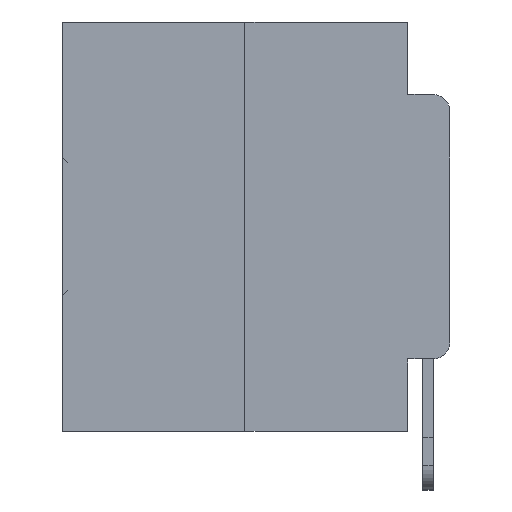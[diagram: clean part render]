
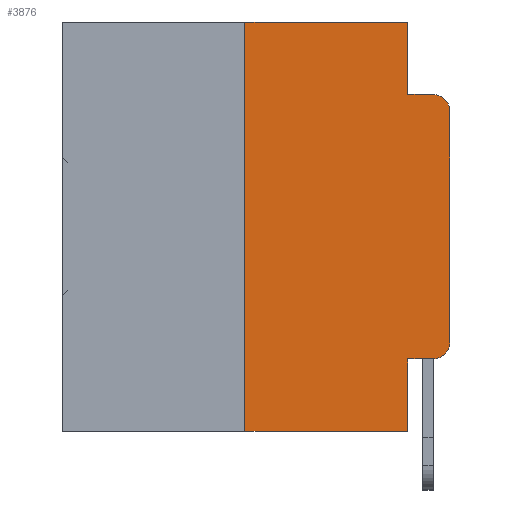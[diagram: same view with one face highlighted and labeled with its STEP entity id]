
A CAD part, left-side view. The second image highlights one B-rep face of the part: STEP entity #3876.
In plain terms, the highlighted planar face has unit normal (-1, 0, 0).
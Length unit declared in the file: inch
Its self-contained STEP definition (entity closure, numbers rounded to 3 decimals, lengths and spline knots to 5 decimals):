
#97 = ORIENTED_EDGE ( 'NONE', *, *, #21235, .T. ) ;
#135 = LINE ( 'NONE', #19567, #6918 ) ;
#479 = ORIENTED_EDGE ( 'NONE', *, *, #22994, .T. ) ;
#750 = EDGE_CURVE ( 'NONE', #11212, #24318, #1622, .T. ) ;
#1141 = VERTEX_POINT ( 'NONE', #31058 ) ;
#1169 = DIRECTION ( 'NONE',  ( -1., 0., 0. ) ) ;
#1191 = FACE_OUTER_BOUND ( 'NONE', #20840, .T. ) ;
#1622 = LINE ( 'NONE', #14650, #21251 ) ;
#2380 = DIRECTION ( 'NONE',  ( -1., 0., 0. ) ) ;
#2948 = EDGE_CURVE ( 'NONE', #11212, #33606, #14081, .T. ) ;
#3170 = EDGE_CURVE ( 'NONE', #8460, #3298, #12047, .T. ) ;
#3298 = VERTEX_POINT ( 'NONE', #5497 ) ;
#3876 = ADVANCED_FACE ( 'NONE', ( #1191 ), #27961, .F. ) ;
#4903 = DIRECTION ( 'NONE',  ( 0., 0., -1. ) ) ;
#5115 = CARTESIAN_POINT ( 'NONE',  ( 0., 0.051, 0. ) ) ;
#5497 = CARTESIAN_POINT ( 'NONE',  ( 0., 0.051, -0.0885 ) ) ;
#5950 = ORIENTED_EDGE ( 'NONE', *, *, #2948, .T. ) ;
#6330 = CARTESIAN_POINT ( 'NONE',  ( 0., 0.25, -0.5 ) ) ;
#6918 = VECTOR ( 'NONE', #27295, 39.37008 ) ;
#7667 = DIRECTION ( 'NONE',  ( 0., 0., 1. ) ) ;
#7864 = VERTEX_POINT ( 'NONE', #27294 ) ;
#7969 = LINE ( 'NONE', #24679, #15649 ) ;
#8308 = CARTESIAN_POINT ( 'NONE',  ( 0., 0.02, -0.4115 ) ) ;
#8460 = VERTEX_POINT ( 'NONE', #30346 ) ;
#8945 = CIRCLE ( 'NONE', #26640, 0.02 ) ;
#9157 = DIRECTION ( 'NONE',  ( 0., -1., 0. ) ) ;
#10724 = CIRCLE ( 'NONE', #29592, 0.02 ) ;
#11212 = VERTEX_POINT ( 'NONE', #6330 ) ;
#12047 = LINE ( 'NONE', #25931, #31865 ) ;
#12480 = CARTESIAN_POINT ( 'NONE',  ( 0., 0.473, 0. ) ) ;
#13298 = LINE ( 'NONE', #26396, #25459 ) ;
#14045 = EDGE_CURVE ( 'NONE', #7864, #20946, #8945, .T. ) ;
#14081 = LINE ( 'NONE', #32479, #21781 ) ;
#14402 = DIRECTION ( 'NONE',  ( 0., -1., 0. ) ) ;
#14650 = CARTESIAN_POINT ( 'NONE',  ( 0., 0.25, 0. ) ) ;
#15064 = DIRECTION ( 'NONE',  ( 0., 0., -1. ) ) ;
#15088 = CARTESIAN_POINT ( 'NONE',  ( 0., 0.25, 0. ) ) ;
#15649 = VECTOR ( 'NONE', #9157, 39.37008 ) ;
#16248 = EDGE_CURVE ( 'NONE', #24318, #8460, #13298, .T. ) ;
#16447 = VECTOR ( 'NONE', #26127, 39.37008 ) ;
#17335 = CARTESIAN_POINT ( 'NONE',  ( 0., 0.02, -0.1085 ) ) ;
#17515 = EDGE_CURVE ( 'NONE', #3298, #20946, #20034, .T. ) ;
#17719 = AXIS2_PLACEMENT_3D ( 'NONE', #12480, #30576, #15064 ) ;
#18067 = LINE ( 'NONE', #5115, #16447 ) ;
#18166 = CARTESIAN_POINT ( 'NONE',  ( 0., 0.051, -0.0885 ) ) ;
#18427 = CARTESIAN_POINT ( 'NONE',  ( 0., 0.02, -0.3915 ) ) ;
#18460 = CARTESIAN_POINT ( 'NONE',  ( 0., 0.02, -0.0885 ) ) ;
#18665 = DIRECTION ( 'NONE',  ( 0., -1., 0. ) ) ;
#18695 = ORIENTED_EDGE ( 'NONE', *, *, #14045, .T. ) ;
#19237 = EDGE_CURVE ( 'NONE', #1141, #7864, #135, .T. ) ;
#19567 = CARTESIAN_POINT ( 'NONE',  ( 0., 0., 0. ) ) ;
#19922 = DIRECTION ( 'NONE',  ( 0., 0., -1. ) ) ;
#19936 = ORIENTED_EDGE ( 'NONE', *, *, #21630, .F. ) ;
#20034 = LINE ( 'NONE', #18166, #32974 ) ;
#20345 = ORIENTED_EDGE ( 'NONE', *, *, #3170, .F. ) ;
#20840 = EDGE_LOOP ( 'NONE', ( #22347, #18695, #32468, #20345, #31275, #26027, #5950, #19936, #97, #479 ) ) ;
#20946 = VERTEX_POINT ( 'NONE', #18460 ) ;
#21038 = DIRECTION ( 'NONE',  ( 0., 0., -1. ) ) ;
#21235 = EDGE_CURVE ( 'NONE', #29143, #23820, #7969, .T. ) ;
#21251 = VECTOR ( 'NONE', #7667, 39.37008 ) ;
#21630 = EDGE_CURVE ( 'NONE', #29143, #33606, #18067, .T. ) ;
#21781 = VECTOR ( 'NONE', #14402, 39.37008 ) ;
#22347 = ORIENTED_EDGE ( 'NONE', *, *, #19237, .T. ) ;
#22994 = EDGE_CURVE ( 'NONE', #23820, #1141, #10724, .T. ) ;
#23820 = VERTEX_POINT ( 'NONE', #8308 ) ;
#24318 = VERTEX_POINT ( 'NONE', #15088 ) ;
#24679 = CARTESIAN_POINT ( 'NONE',  ( 0., 0.051, -0.4115 ) ) ;
#25459 = VECTOR ( 'NONE', #18665, 39.37008 ) ;
#25931 = CARTESIAN_POINT ( 'NONE',  ( 0., 0.051, 0. ) ) ;
#26027 = ORIENTED_EDGE ( 'NONE', *, *, #750, .F. ) ;
#26127 = DIRECTION ( 'NONE',  ( 0., 0., -1. ) ) ;
#26396 = CARTESIAN_POINT ( 'NONE',  ( 0., 0.473, 0. ) ) ;
#26640 = AXIS2_PLACEMENT_3D ( 'NONE', #17335, #1169, #19922 ) ;
#27294 = CARTESIAN_POINT ( 'NONE',  ( 0., 0., -0.1085 ) ) ;
#27295 = DIRECTION ( 'NONE',  ( 0., 0., 1. ) ) ;
#27961 = PLANE ( 'NONE',  #17719 ) ;
#29143 = VERTEX_POINT ( 'NONE', #29587 ) ;
#29587 = CARTESIAN_POINT ( 'NONE',  ( 0., 0.051, -0.4115 ) ) ;
#29592 = AXIS2_PLACEMENT_3D ( 'NONE', #18427, #2380, #21038 ) ;
#30346 = CARTESIAN_POINT ( 'NONE',  ( 0., 0.051, 0. ) ) ;
#30576 = DIRECTION ( 'NONE',  ( 1., 0., 0. ) ) ;
#31058 = CARTESIAN_POINT ( 'NONE',  ( 0., 0., -0.3915 ) ) ;
#31191 = DIRECTION ( 'NONE',  ( 0., -1., 0. ) ) ;
#31275 = ORIENTED_EDGE ( 'NONE', *, *, #16248, .F. ) ;
#31865 = VECTOR ( 'NONE', #4903, 39.37008 ) ;
#32468 = ORIENTED_EDGE ( 'NONE', *, *, #17515, .F. ) ;
#32479 = CARTESIAN_POINT ( 'NONE',  ( 0., 0.473, -0.5 ) ) ;
#32974 = VECTOR ( 'NONE', #31191, 39.37008 ) ;
#33066 = CARTESIAN_POINT ( 'NONE',  ( 0., 0.051, -0.5 ) ) ;
#33606 = VERTEX_POINT ( 'NONE', #33066 ) ;
